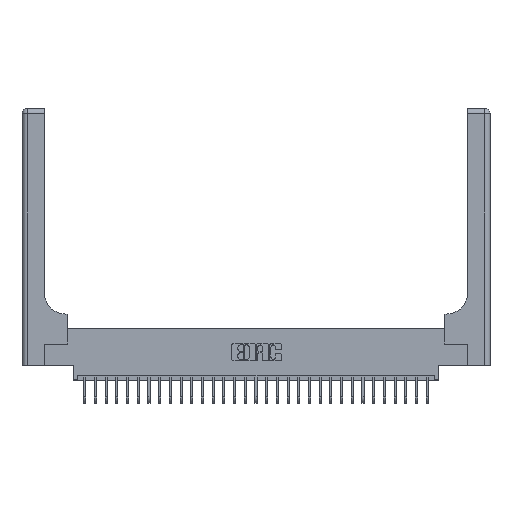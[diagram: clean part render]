
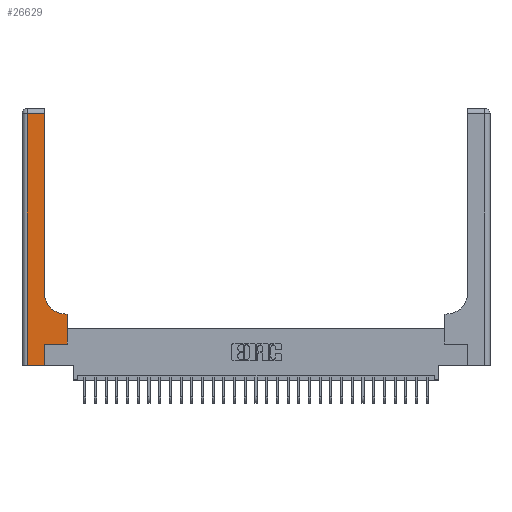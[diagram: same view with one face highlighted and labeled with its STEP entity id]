
A CAD part, top view. The second image highlights one B-rep face of the part: STEP entity #26629.
In plain terms, the highlighted planar face has unit normal (0, 0, 1).
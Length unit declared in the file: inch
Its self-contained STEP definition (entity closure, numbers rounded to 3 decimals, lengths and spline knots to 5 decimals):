
#204 = VECTOR ( 'NONE', #28913, 39.37008 ) ;
#316 = LINE ( 'NONE', #28378, #8892 ) ;
#672 = VERTEX_POINT ( 'NONE', #29831 ) ;
#858 = ORIENTED_EDGE ( 'NONE', *, *, #1312, .T. ) ;
#1109 = EDGE_CURVE ( 'NONE', #3572, #13805, #16121, .T. ) ;
#1247 = VECTOR ( 'NONE', #25478, 39.37008 ) ;
#1312 = EDGE_CURVE ( 'NONE', #14368, #3572, #12545, .T. ) ;
#1794 = VERTEX_POINT ( 'NONE', #8444 ) ;
#1933 = CARTESIAN_POINT ( 'NONE',  ( 0.51, 0.6, 0.37 ) ) ;
#2039 = EDGE_CURVE ( 'NONE', #21318, #3976, #316, .T. ) ;
#3238 = VECTOR ( 'NONE', #4630, 39.37008 ) ;
#3572 = VERTEX_POINT ( 'NONE', #11162 ) ;
#3669 = LINE ( 'NONE', #12408, #19850 ) ;
#3976 = VERTEX_POINT ( 'NONE', #15275 ) ;
#4471 = CARTESIAN_POINT ( 'NONE',  ( 0.06, 3., 0.37 ) ) ;
#4630 = DIRECTION ( 'NONE',  ( 0., 1., 0. ) ) ;
#6579 = ORIENTED_EDGE ( 'NONE', *, *, #1109, .T. ) ;
#6651 = ORIENTED_EDGE ( 'NONE', *, *, #11619, .T. ) ;
#7483 = EDGE_LOOP ( 'NONE', ( #6579, #23657, #20469, #19541, #6651, #28762, #17147, #11976, #858 ) ) ;
#7883 = DIRECTION ( 'NONE',  ( 0., 0., -1. ) ) ;
#8444 = CARTESIAN_POINT ( 'NONE',  ( 0.265, 0.25, 0.37 ) ) ;
#8892 = VECTOR ( 'NONE', #14253, 39.37008 ) ;
#9632 = CARTESIAN_POINT ( 'NONE',  ( 0.265, 0., 0.37 ) ) ;
#9724 = EDGE_CURVE ( 'NONE', #672, #12224, #19563, .T. ) ;
#10173 = FACE_OUTER_BOUND ( 'NONE', #7483, .T. ) ;
#10331 = CARTESIAN_POINT ( 'NONE',  ( 0., 0., 0.37 ) ) ;
#10537 = EDGE_CURVE ( 'NONE', #3976, #14368, #3669, .T. ) ;
#11007 = CARTESIAN_POINT ( 'NONE',  ( 0.51, 0.85, 0.37 ) ) ;
#11162 = CARTESIAN_POINT ( 'NONE',  ( 0.26, 0.85, 0.37 ) ) ;
#11200 = LINE ( 'NONE', #4471, #28050 ) ;
#11619 = EDGE_CURVE ( 'NONE', #12224, #1794, #18599, .T. ) ;
#11976 = ORIENTED_EDGE ( 'NONE', *, *, #10537, .T. ) ;
#12138 = CARTESIAN_POINT ( 'NONE',  ( 0., 2.94, 0.37 ) ) ;
#12202 = VECTOR ( 'NONE', #17954, 39.37008 ) ;
#12224 = VERTEX_POINT ( 'NONE', #9632 ) ;
#12408 = CARTESIAN_POINT ( 'NONE',  ( 0.26, 0.6, 0.37 ) ) ;
#12531 = VERTEX_POINT ( 'NONE', #22477 ) ;
#12545 = CIRCLE ( 'NONE', #23816, 0.25 ) ;
#12741 = AXIS2_PLACEMENT_3D ( 'NONE', #24725, #7883, #14926 ) ;
#13805 = VERTEX_POINT ( 'NONE', #22634 ) ;
#14253 = DIRECTION ( 'NONE',  ( 0., 1., 0. ) ) ;
#14368 = VERTEX_POINT ( 'NONE', #1933 ) ;
#14926 = DIRECTION ( 'NONE',  ( -1., 0., 0. ) ) ;
#15232 = PLANE ( 'NONE',  #12741 ) ;
#15275 = CARTESIAN_POINT ( 'NONE',  ( 0.528, 0.6, 0.37 ) ) ;
#16121 = LINE ( 'NONE', #27627, #1247 ) ;
#17147 = ORIENTED_EDGE ( 'NONE', *, *, #2039, .T. ) ;
#17954 = DIRECTION ( 'NONE',  ( 1., 0., 0. ) ) ;
#18599 = LINE ( 'NONE', #27947, #3238 ) ;
#19241 = EDGE_CURVE ( 'NONE', #1794, #21318, #20100, .T. ) ;
#19541 = ORIENTED_EDGE ( 'NONE', *, *, #9724, .T. ) ;
#19563 = LINE ( 'NONE', #10331, #204 ) ;
#19584 = VECTOR ( 'NONE', #28410, 39.37008 ) ;
#19786 = DIRECTION ( 'NONE',  ( -1., 0., 0. ) ) ;
#19850 = VECTOR ( 'NONE', #19786, 39.37008 ) ;
#20100 = LINE ( 'NONE', #26844, #12202 ) ;
#20469 = ORIENTED_EDGE ( 'NONE', *, *, #28399, .T. ) ;
#21318 = VERTEX_POINT ( 'NONE', #26478 ) ;
#22477 = CARTESIAN_POINT ( 'NONE',  ( 0.06, 2.94, 0.37 ) ) ;
#22634 = CARTESIAN_POINT ( 'NONE',  ( 0.26, 2.94, 0.37 ) ) ;
#23657 = ORIENTED_EDGE ( 'NONE', *, *, #23769, .T. ) ;
#23769 = EDGE_CURVE ( 'NONE', #13805, #12531, #28265, .T. ) ;
#23816 = AXIS2_PLACEMENT_3D ( 'NONE', #11007, #24648, #24960 ) ;
#24648 = DIRECTION ( 'NONE',  ( 0., 0., -1. ) ) ;
#24725 = CARTESIAN_POINT ( 'NONE',  ( 0., 3., 0.37 ) ) ;
#24960 = DIRECTION ( 'NONE',  ( 1., 0., 0. ) ) ;
#25478 = DIRECTION ( 'NONE',  ( 0., 1., 0. ) ) ;
#26478 = CARTESIAN_POINT ( 'NONE',  ( 0.528, 0.25, 0.37 ) ) ;
#26629 = ADVANCED_FACE ( 'NONE', ( #10173 ), #15232, .F. ) ;
#26844 = CARTESIAN_POINT ( 'NONE',  ( 0.265, 0.25, 0.37 ) ) ;
#27465 = DIRECTION ( 'NONE',  ( 0., -1., 0. ) ) ;
#27627 = CARTESIAN_POINT ( 'NONE',  ( 0.26, 3., 0.37 ) ) ;
#27947 = CARTESIAN_POINT ( 'NONE',  ( 0.265, 0., 0.37 ) ) ;
#28050 = VECTOR ( 'NONE', #27465, 39.37008 ) ;
#28265 = LINE ( 'NONE', #12138, #19584 ) ;
#28378 = CARTESIAN_POINT ( 'NONE',  ( 0.528, 0.25, 0.37 ) ) ;
#28399 = EDGE_CURVE ( 'NONE', #12531, #672, #11200, .T. ) ;
#28410 = DIRECTION ( 'NONE',  ( -1., 0., 0. ) ) ;
#28762 = ORIENTED_EDGE ( 'NONE', *, *, #19241, .T. ) ;
#28913 = DIRECTION ( 'NONE',  ( 1., 0., 0. ) ) ;
#29831 = CARTESIAN_POINT ( 'NONE',  ( 0.06, 0., 0.37 ) ) ;
